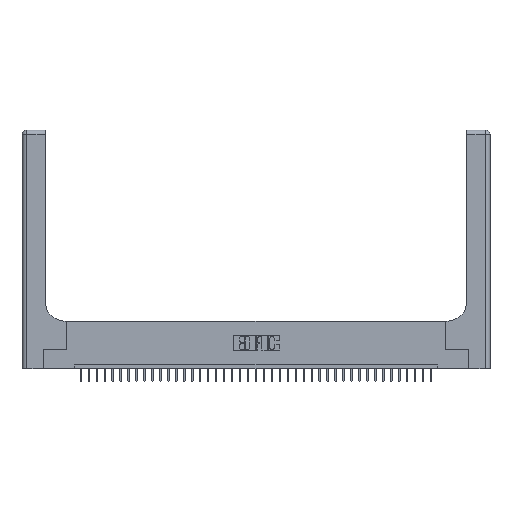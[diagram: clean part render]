
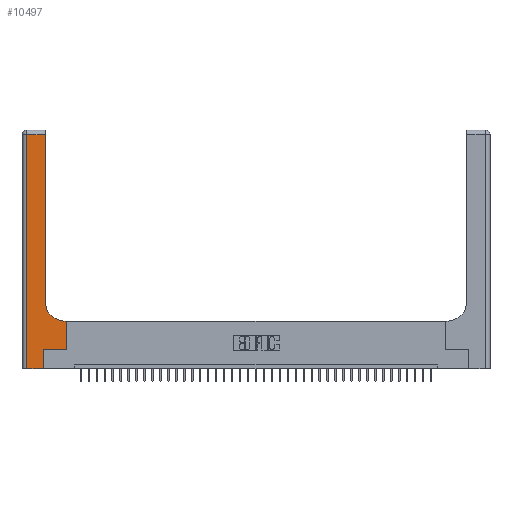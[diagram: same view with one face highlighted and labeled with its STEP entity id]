
A CAD part, top view. The second image highlights one B-rep face of the part: STEP entity #10497.
In plain terms, the highlighted planar face has unit normal (0, 0, 1).
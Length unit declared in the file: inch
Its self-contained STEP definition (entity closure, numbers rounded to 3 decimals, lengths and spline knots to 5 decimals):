
#374 = DIRECTION ( 'NONE',  ( -1., 0., 0. ) ) ;
#758 = CARTESIAN_POINT ( 'NONE',  ( 0.5415, 0.6, 0.37 ) ) ;
#826 = CARTESIAN_POINT ( 'NONE',  ( 0.2915, 0.85, 0.37 ) ) ;
#1106 = DIRECTION ( 'NONE',  ( 1., 0., 0. ) ) ;
#1128 = CARTESIAN_POINT ( 'NONE',  ( 0.269, 0.25, 0.37 ) ) ;
#1370 = DIRECTION ( 'NONE',  ( 0., 0., -1. ) ) ;
#1535 = DIRECTION ( 'NONE',  ( 1., 0., 0. ) ) ;
#2628 = EDGE_CURVE ( 'NONE', #33916, #17544, #37829, .T. ) ;
#3097 = VECTOR ( 'NONE', #17241, 39.37008 ) ;
#4048 = EDGE_CURVE ( 'NONE', #16073, #33916, #24544, .T. ) ;
#4535 = CARTESIAN_POINT ( 'NONE',  ( 0., 0., 0.37 ) ) ;
#4777 = ORIENTED_EDGE ( 'NONE', *, *, #38107, .T. ) ;
#6507 = LINE ( 'NONE', #1128, #10295 ) ;
#6557 = CARTESIAN_POINT ( 'NONE',  ( 0.269, 0., 0.37 ) ) ;
#6880 = ORIENTED_EDGE ( 'NONE', *, *, #4048, .T. ) ;
#7189 = LINE ( 'NONE', #4535, #38078 ) ;
#8825 = EDGE_LOOP ( 'NONE', ( #20499, #14804, #23310, #24039, #38304, #26265, #4777, #24309, #6880 ) ) ;
#9100 = FACE_OUTER_BOUND ( 'NONE', #8825, .T. ) ;
#9954 = CARTESIAN_POINT ( 'NONE',  ( 0.2915, 0.6, 0.37 ) ) ;
#10215 = CARTESIAN_POINT ( 'NONE',  ( 0., 3., 0.37 ) ) ;
#10295 = VECTOR ( 'NONE', #1535, 39.37008 ) ;
#10497 = ADVANCED_FACE ( 'NONE', ( #9100 ), #19075, .F. ) ;
#11368 = VECTOR ( 'NONE', #33782, 39.37008 ) ;
#11620 = VERTEX_POINT ( 'NONE', #34153 ) ;
#12456 = EDGE_CURVE ( 'NONE', #11620, #16073, #37465, .T. ) ;
#12836 = CARTESIAN_POINT ( 'NONE',  ( 0.5585, 0.25, 0.37 ) ) ;
#13208 = DIRECTION ( 'NONE',  ( 0., 0., -1. ) ) ;
#13467 = DIRECTION ( 'NONE',  ( -1., 0., 0. ) ) ;
#13496 = VERTEX_POINT ( 'NONE', #36440 ) ;
#13902 = VERTEX_POINT ( 'NONE', #12836 ) ;
#13949 = VECTOR ( 'NONE', #22112, 39.37008 ) ;
#14804 = ORIENTED_EDGE ( 'NONE', *, *, #19888, .T. ) ;
#16073 = VERTEX_POINT ( 'NONE', #758 ) ;
#17241 = DIRECTION ( 'NONE',  ( 0., -1., 0. ) ) ;
#17544 = VERTEX_POINT ( 'NONE', #28630 ) ;
#18207 = CARTESIAN_POINT ( 'NONE',  ( 0.269, 0.25, 0.37 ) ) ;
#19075 = PLANE ( 'NONE',  #36986 ) ;
#19109 = DIRECTION ( 'NONE',  ( 0., 1., 0. ) ) ;
#19503 = CARTESIAN_POINT ( 'NONE',  ( 0.5415, 0.85, 0.37 ) ) ;
#19888 = EDGE_CURVE ( 'NONE', #17544, #24035, #37433, .T. ) ;
#20499 = ORIENTED_EDGE ( 'NONE', *, *, #2628, .T. ) ;
#20649 = LINE ( 'NONE', #31525, #33291 ) ;
#22112 = DIRECTION ( 'NONE',  ( 0., 1., 0. ) ) ;
#22396 = DIRECTION ( 'NONE',  ( 1., 0., 0. ) ) ;
#23310 = ORIENTED_EDGE ( 'NONE', *, *, #32219, .T. ) ;
#24035 = VERTEX_POINT ( 'NONE', #38281 ) ;
#24039 = ORIENTED_EDGE ( 'NONE', *, *, #24124, .T. ) ;
#24124 = EDGE_CURVE ( 'NONE', #13496, #31243, #7189, .T. ) ;
#24309 = ORIENTED_EDGE ( 'NONE', *, *, #12456, .T. ) ;
#24544 = CIRCLE ( 'NONE', #30238, 0.25 ) ;
#25228 = VECTOR ( 'NONE', #36467, 39.37008 ) ;
#26265 = ORIENTED_EDGE ( 'NONE', *, *, #30013, .T. ) ;
#26416 = VERTEX_POINT ( 'NONE', #18207 ) ;
#27045 = CARTESIAN_POINT ( 'NONE',  ( 0.269, 0., 0.37 ) ) ;
#28500 = VECTOR ( 'NONE', #374, 39.37008 ) ;
#28602 = CARTESIAN_POINT ( 'NONE',  ( 0.06, 3., 0.37 ) ) ;
#28630 = CARTESIAN_POINT ( 'NONE',  ( 0.2915, 2.94, 0.37 ) ) ;
#29542 = LINE ( 'NONE', #6557, #11368 ) ;
#30013 = EDGE_CURVE ( 'NONE', #26416, #13902, #6507, .T. ) ;
#30238 = AXIS2_PLACEMENT_3D ( 'NONE', #19503, #1370, #1106 ) ;
#31243 = VERTEX_POINT ( 'NONE', #27045 ) ;
#31525 = CARTESIAN_POINT ( 'NONE',  ( 0.5585, 0.25, 0.37 ) ) ;
#32091 = LINE ( 'NONE', #28602, #3097 ) ;
#32219 = EDGE_CURVE ( 'NONE', #24035, #13496, #32091, .T. ) ;
#33291 = VECTOR ( 'NONE', #19109, 39.37008 ) ;
#33782 = DIRECTION ( 'NONE',  ( 0., 1., 0. ) ) ;
#33916 = VERTEX_POINT ( 'NONE', #826 ) ;
#34153 = CARTESIAN_POINT ( 'NONE',  ( 0.5585, 0.6, 0.37 ) ) ;
#36440 = CARTESIAN_POINT ( 'NONE',  ( 0.06, 0., 0.37 ) ) ;
#36467 = DIRECTION ( 'NONE',  ( -1., 0., 0. ) ) ;
#36986 = AXIS2_PLACEMENT_3D ( 'NONE', #10215, #13208, #13467 ) ;
#37329 = CARTESIAN_POINT ( 'NONE',  ( 0.2915, 3., 0.37 ) ) ;
#37433 = LINE ( 'NONE', #38221, #28500 ) ;
#37465 = LINE ( 'NONE', #9954, #25228 ) ;
#37829 = LINE ( 'NONE', #37329, #13949 ) ;
#38008 = EDGE_CURVE ( 'NONE', #31243, #26416, #29542, .T. ) ;
#38078 = VECTOR ( 'NONE', #22396, 39.37008 ) ;
#38107 = EDGE_CURVE ( 'NONE', #13902, #11620, #20649, .T. ) ;
#38221 = CARTESIAN_POINT ( 'NONE',  ( 0., 2.94, 0.37 ) ) ;
#38281 = CARTESIAN_POINT ( 'NONE',  ( 0.06, 2.94, 0.37 ) ) ;
#38304 = ORIENTED_EDGE ( 'NONE', *, *, #38008, .T. ) ;
